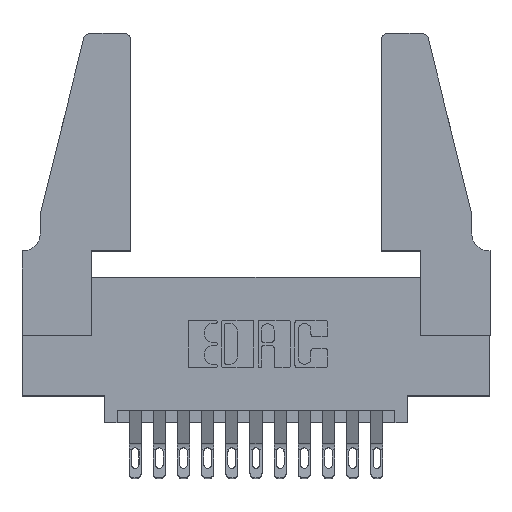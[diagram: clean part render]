
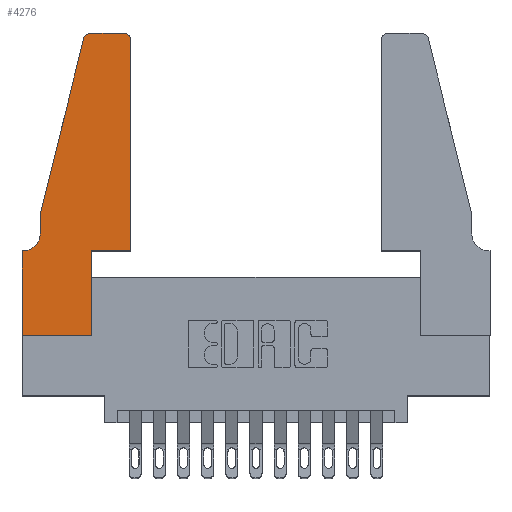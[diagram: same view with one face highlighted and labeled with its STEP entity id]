
A CAD part, top view. The second image highlights one B-rep face of the part: STEP entity #4276.
In plain terms, the highlighted planar face has unit normal (0, 0, 1).
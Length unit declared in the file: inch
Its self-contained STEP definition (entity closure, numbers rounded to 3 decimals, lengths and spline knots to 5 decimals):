
#248 = CARTESIAN_POINT ( 'NONE',  ( 0.2865, 0.35, 0.37 ) ) ;
#338 = EDGE_LOOP ( 'NONE', ( #1283, #7633, #5661, #12852, #8990, #1180, #2056, #1983, #7428, #15184, #10894, #3108 ) ) ;
#399 = DIRECTION ( 'NONE',  ( 1., 0., 0. ) ) ;
#475 = CARTESIAN_POINT ( 'NONE',  ( 0., 0., 0.37 ) ) ;
#660 = LINE ( 'NONE', #475, #3615 ) ;
#678 = EDGE_CURVE ( 'NONE', #5893, #7045, #660, .T. ) ;
#934 = EDGE_CURVE ( 'NONE', #11188, #12735, #13633, .T. ) ;
#954 = VERTEX_POINT ( 'NONE', #4943 ) ;
#1138 = DIRECTION ( 'NONE',  ( 0., -1., 0. ) ) ;
#1180 = ORIENTED_EDGE ( 'NONE', *, *, #5142, .T. ) ;
#1228 = DIRECTION ( 'NONE',  ( 0., 0., -1. ) ) ;
#1283 = ORIENTED_EDGE ( 'NONE', *, *, #8903, .T. ) ;
#1450 = EDGE_CURVE ( 'NONE', #7045, #10923, #3408, .T. ) ;
#1605 = CIRCLE ( 'NONE', #9022, 0.03 ) ;
#1983 = ORIENTED_EDGE ( 'NONE', *, *, #678, .T. ) ;
#2056 = ORIENTED_EDGE ( 'NONE', *, *, #2330, .T. ) ;
#2250 = VECTOR ( 'NONE', #8612, 39.37008 ) ;
#2288 = VERTEX_POINT ( 'NONE', #4738 ) ;
#2330 = EDGE_CURVE ( 'NONE', #954, #5893, #10904, .T. ) ;
#2437 = DIRECTION ( 'NONE',  ( -1., 0., 0. ) ) ;
#2649 = VERTEX_POINT ( 'NONE', #12508 ) ;
#3108 = ORIENTED_EDGE ( 'NONE', *, *, #7439, .T. ) ;
#3114 = AXIS2_PLACEMENT_3D ( 'NONE', #8244, #5915, #14093 ) ;
#3187 = VECTOR ( 'NONE', #8257, 39.37008 ) ;
#3408 = LINE ( 'NONE', #10495, #9080 ) ;
#3434 = DIRECTION ( 'NONE',  ( 0., 0., 1. ) ) ;
#3615 = VECTOR ( 'NONE', #399, 39.37008 ) ;
#3643 = CARTESIAN_POINT ( 'NONE',  ( 0.4505, 0.35, 0.37 ) ) ;
#3819 = CARTESIAN_POINT ( 'NONE',  ( 0.2865, 0., 0.37 ) ) ;
#3908 = VECTOR ( 'NONE', #2437, 39.37008 ) ;
#4276 = ADVANCED_FACE ( 'NONE', ( #9563 ), #12944, .T. ) ;
#4302 = LINE ( 'NONE', #14302, #3908 ) ;
#4382 = EDGE_CURVE ( 'NONE', #14469, #2288, #11602, .T. ) ;
#4484 = CARTESIAN_POINT ( 'NONE',  ( 0.25487, 1.22718, 0.37 ) ) ;
#4656 = AXIS2_PLACEMENT_3D ( 'NONE', #8550, #1228, #9737 ) ;
#4738 = CARTESIAN_POINT ( 'NONE',  ( 0.4505, 1.22, 0.37 ) ) ;
#4943 = CARTESIAN_POINT ( 'NONE',  ( 0., 0.35, 0.37 ) ) ;
#5142 = EDGE_CURVE ( 'NONE', #14306, #954, #8917, .T. ) ;
#5438 = CARTESIAN_POINT ( 'NONE',  ( 0.0755, 0.5, 0.37 ) ) ;
#5476 = DIRECTION ( 'NONE',  ( 0., 0., 1. ) ) ;
#5661 = ORIENTED_EDGE ( 'NONE', *, *, #5875, .T. ) ;
#5875 = EDGE_CURVE ( 'NONE', #6787, #11188, #8699, .T. ) ;
#5893 = VERTEX_POINT ( 'NONE', #12116 ) ;
#5915 = DIRECTION ( 'NONE',  ( 0., 0., 1. ) ) ;
#6443 = LINE ( 'NONE', #8313, #3187 ) ;
#6787 = VERTEX_POINT ( 'NONE', #4484 ) ;
#6895 = EDGE_CURVE ( 'NONE', #10923, #14469, #6443, .T. ) ;
#7045 = VERTEX_POINT ( 'NONE', #3819 ) ;
#7428 = ORIENTED_EDGE ( 'NONE', *, *, #1450, .T. ) ;
#7439 = EDGE_CURVE ( 'NONE', #2288, #10127, #1605, .T. ) ;
#7633 = ORIENTED_EDGE ( 'NONE', *, *, #15430, .T. ) ;
#7652 = CARTESIAN_POINT ( 'NONE',  ( 0.0755, 0.35, 0.37 ) ) ;
#8244 = CARTESIAN_POINT ( 'NONE',  ( 0., 0.35, 0.37 ) ) ;
#8257 = DIRECTION ( 'NONE',  ( 1., 0., 0. ) ) ;
#8313 = CARTESIAN_POINT ( 'NONE',  ( 0.4505, 0.35, 0.37 ) ) ;
#8405 = CARTESIAN_POINT ( 'NONE',  ( 0., 0., 0.37 ) ) ;
#8550 = CARTESIAN_POINT ( 'NONE',  ( 0.0055, 0.42, 0.37 ) ) ;
#8612 = DIRECTION ( 'NONE',  ( -0.239, -0.971, 0. ) ) ;
#8699 = LINE ( 'NONE', #9795, #2250 ) ;
#8903 = EDGE_CURVE ( 'NONE', #10127, #2649, #4302, .T. ) ;
#8917 = LINE ( 'NONE', #7652, #14676 ) ;
#8990 = ORIENTED_EDGE ( 'NONE', *, *, #10214, .T. ) ;
#9022 = AXIS2_PLACEMENT_3D ( 'NONE', #10629, #3434, #11824 ) ;
#9065 = CARTESIAN_POINT ( 'NONE',  ( 0.0755, 0.42, 0.37 ) ) ;
#9080 = VECTOR ( 'NONE', #10441, 39.37008 ) ;
#9563 = FACE_OUTER_BOUND ( 'NONE', #338, .T. ) ;
#9737 = DIRECTION ( 'NONE',  ( -1., 0., 0. ) ) ;
#9795 = CARTESIAN_POINT ( 'NONE',  ( 0.0755, 0.5, 0.37 ) ) ;
#10127 = VERTEX_POINT ( 'NONE', #10720 ) ;
#10214 = EDGE_CURVE ( 'NONE', #12735, #14306, #13687, .T. ) ;
#10340 = CARTESIAN_POINT ( 'NONE',  ( 0.0055, 0.35, 0.37 ) ) ;
#10441 = DIRECTION ( 'NONE',  ( 0., 1., 0. ) ) ;
#10495 = CARTESIAN_POINT ( 'NONE',  ( 0.2865, 0.35, 0.37 ) ) ;
#10629 = CARTESIAN_POINT ( 'NONE',  ( 0.4205, 1.22, 0.37 ) ) ;
#10720 = CARTESIAN_POINT ( 'NONE',  ( 0.4205, 1.25, 0.37 ) ) ;
#10801 = AXIS2_PLACEMENT_3D ( 'NONE', #12538, #5476, #13684 ) ;
#10894 = ORIENTED_EDGE ( 'NONE', *, *, #4382, .T. ) ;
#10904 = LINE ( 'NONE', #8405, #12872 ) ;
#10923 = VERTEX_POINT ( 'NONE', #248 ) ;
#11188 = VERTEX_POINT ( 'NONE', #15165 ) ;
#11194 = DIRECTION ( 'NONE',  ( -1., 0., 0. ) ) ;
#11602 = LINE ( 'NONE', #3643, #14252 ) ;
#11824 = DIRECTION ( 'NONE',  ( 1., 0., 0. ) ) ;
#12116 = CARTESIAN_POINT ( 'NONE',  ( 0., 0., 0.37 ) ) ;
#12508 = CARTESIAN_POINT ( 'NONE',  ( 0.284, 1.25, 0.37 ) ) ;
#12538 = CARTESIAN_POINT ( 'NONE',  ( 0.284, 1.22, 0.37 ) ) ;
#12563 = VECTOR ( 'NONE', #1138, 39.37008 ) ;
#12735 = VERTEX_POINT ( 'NONE', #9065 ) ;
#12852 = ORIENTED_EDGE ( 'NONE', *, *, #934, .T. ) ;
#12872 = VECTOR ( 'NONE', #14179, 39.37008 ) ;
#12944 = PLANE ( 'NONE',  #3114 ) ;
#13142 = DIRECTION ( 'NONE',  ( 0., 1., 0. ) ) ;
#13633 = LINE ( 'NONE', #5438, #12563 ) ;
#13684 = DIRECTION ( 'NONE',  ( 1., 0., 0. ) ) ;
#13687 = CIRCLE ( 'NONE', #4656, 0.07 ) ;
#14052 = CARTESIAN_POINT ( 'NONE',  ( 0.4505, 0.35, 0.37 ) ) ;
#14088 = CIRCLE ( 'NONE', #10801, 0.03 ) ;
#14093 = DIRECTION ( 'NONE',  ( 1., 0., 0. ) ) ;
#14179 = DIRECTION ( 'NONE',  ( 0., -1., 0. ) ) ;
#14252 = VECTOR ( 'NONE', #13142, 39.37008 ) ;
#14302 = CARTESIAN_POINT ( 'NONE',  ( 0.2605, 1.25, 0.37 ) ) ;
#14306 = VERTEX_POINT ( 'NONE', #10340 ) ;
#14469 = VERTEX_POINT ( 'NONE', #14052 ) ;
#14676 = VECTOR ( 'NONE', #11194, 39.37008 ) ;
#15165 = CARTESIAN_POINT ( 'NONE',  ( 0.0755, 0.5, 0.37 ) ) ;
#15184 = ORIENTED_EDGE ( 'NONE', *, *, #6895, .T. ) ;
#15430 = EDGE_CURVE ( 'NONE', #2649, #6787, #14088, .T. ) ;
